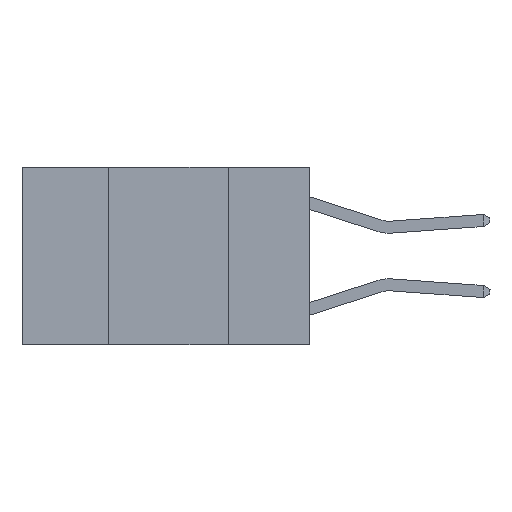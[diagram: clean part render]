
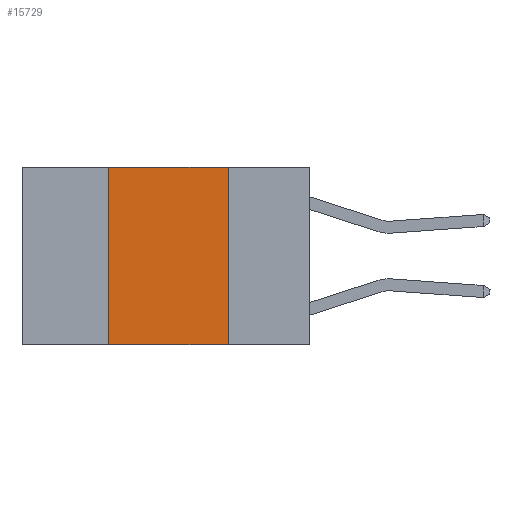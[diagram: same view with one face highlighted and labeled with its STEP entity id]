
A CAD part, left-side view. The second image highlights one B-rep face of the part: STEP entity #15729.
In plain terms, the highlighted planar face has unit normal (-1, 0, 0).
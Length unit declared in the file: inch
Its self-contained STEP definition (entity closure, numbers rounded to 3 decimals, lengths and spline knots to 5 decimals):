
#110 = CARTESIAN_POINT ( 'NONE',  ( 0., 0.6, -0.37 ) ) ;
#473 = FACE_OUTER_BOUND ( 'NONE', #9539, .T. ) ;
#618 = VERTEX_POINT ( 'NONE', #16413 ) ;
#1146 = CARTESIAN_POINT ( 'NONE',  ( 0., 0.42, 0. ) ) ;
#2375 = PLANE ( 'NONE',  #14039 ) ;
#2439 = DIRECTION ( 'NONE',  ( 0., 0., -1. ) ) ;
#3284 = DIRECTION ( 'NONE',  ( 0., 0., -1. ) ) ;
#3293 = VERTEX_POINT ( 'NONE', #17856 ) ;
#3347 = CARTESIAN_POINT ( 'NONE',  ( 0., 0.17, 0. ) ) ;
#3699 = CARTESIAN_POINT ( 'NONE',  ( 0., 0.17, -0.37 ) ) ;
#5880 = DIRECTION ( 'NONE',  ( 0., 0., 1. ) ) ;
#7742 = EDGE_CURVE ( 'NONE', #618, #3293, #14077, .T. ) ;
#8164 = CARTESIAN_POINT ( 'NONE',  ( 0., 0.17, 0. ) ) ;
#8665 = CARTESIAN_POINT ( 'NONE',  ( 0., 0.6, 0. ) ) ;
#8805 = ORIENTED_EDGE ( 'NONE', *, *, #7742, .F. ) ;
#8911 = LINE ( 'NONE', #3347, #13032 ) ;
#8984 = VECTOR ( 'NONE', #17181, 39.37008 ) ;
#9460 = LINE ( 'NONE', #110, #8984 ) ;
#9539 = EDGE_LOOP ( 'NONE', ( #10497, #15083, #8805, #19352 ) ) ;
#9563 = EDGE_CURVE ( 'NONE', #3293, #11223, #15757, .T. ) ;
#9949 = VECTOR ( 'NONE', #5880, 39.37008 ) ;
#10497 = ORIENTED_EDGE ( 'NONE', *, *, #12975, .F. ) ;
#11130 = EDGE_CURVE ( 'NONE', #618, #13138, #9460, .T. ) ;
#11223 = VERTEX_POINT ( 'NONE', #8164 ) ;
#11790 = DIRECTION ( 'NONE',  ( 1., 0., 0. ) ) ;
#12177 = VECTOR ( 'NONE', #16722, 39.37008 ) ;
#12975 = EDGE_CURVE ( 'NONE', #11223, #13138, #8911, .T. ) ;
#13032 = VECTOR ( 'NONE', #3284, 39.37008 ) ;
#13138 = VERTEX_POINT ( 'NONE', #3699 ) ;
#14039 = AXIS2_PLACEMENT_3D ( 'NONE', #8665, #11790, #2439 ) ;
#14077 = LINE ( 'NONE', #1146, #9949 ) ;
#15083 = ORIENTED_EDGE ( 'NONE', *, *, #9563, .F. ) ;
#15729 = ADVANCED_FACE ( 'NONE', ( #473 ), #2375, .F. ) ;
#15757 = LINE ( 'NONE', #16790, #12177 ) ;
#16413 = CARTESIAN_POINT ( 'NONE',  ( 0., 0.42, -0.37 ) ) ;
#16722 = DIRECTION ( 'NONE',  ( 0., -1., 0. ) ) ;
#16790 = CARTESIAN_POINT ( 'NONE',  ( 0., 0.6, 0. ) ) ;
#17181 = DIRECTION ( 'NONE',  ( 0., -1., 0. ) ) ;
#17856 = CARTESIAN_POINT ( 'NONE',  ( 0., 0.42, 0. ) ) ;
#19352 = ORIENTED_EDGE ( 'NONE', *, *, #11130, .T. ) ;
